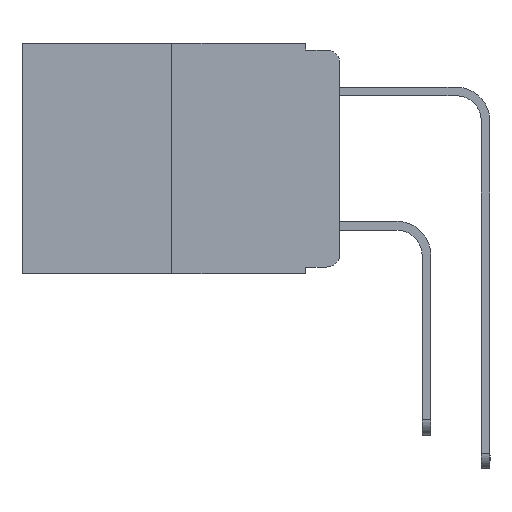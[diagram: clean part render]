
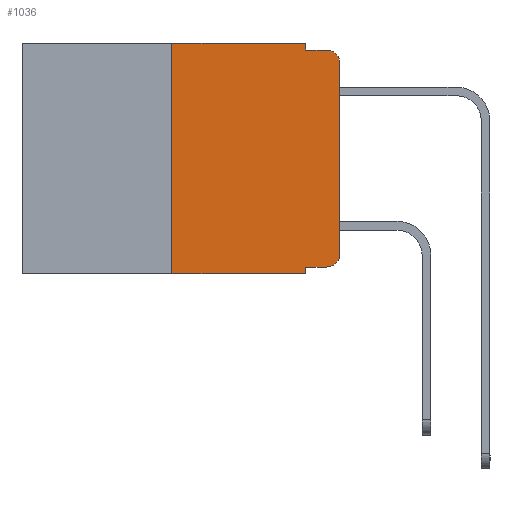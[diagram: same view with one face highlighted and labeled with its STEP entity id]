
A CAD part, left-side view. The second image highlights one B-rep face of the part: STEP entity #1036.
In plain terms, the highlighted planar face has unit normal (-1, 0, 0).
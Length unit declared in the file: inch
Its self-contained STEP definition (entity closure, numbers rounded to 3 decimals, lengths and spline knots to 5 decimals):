
#616 = ORIENTED_EDGE ( 'NONE', *, *, #22179, .F. ) ;
#884 = DIRECTION ( 'NONE',  ( 1., 0., 0. ) ) ;
#899 = LINE ( 'NONE', #18932, #20484 ) ;
#1036 = ADVANCED_FACE ( 'NONE', ( #2227 ), #2343, .F. ) ;
#1253 = DIRECTION ( 'NONE',  ( 0., -1., 0. ) ) ;
#1555 = ORIENTED_EDGE ( 'NONE', *, *, #3962, .F. ) ;
#1661 = CARTESIAN_POINT ( 'NONE',  ( 0., 0.473, 0. ) ) ;
#1679 = CARTESIAN_POINT ( 'NONE',  ( 0., 0., 0. ) ) ;
#1693 = CARTESIAN_POINT ( 'NONE',  ( 0., 0., -0.313 ) ) ;
#2227 = FACE_OUTER_BOUND ( 'NONE', #21097, .T. ) ;
#2343 = PLANE ( 'NONE',  #21999 ) ;
#2802 = CARTESIAN_POINT ( 'NONE',  ( 0., 0.051, -0.343 ) ) ;
#2828 = DIRECTION ( 'NONE',  ( 0., 0., -1. ) ) ;
#3444 = DIRECTION ( 'NONE',  ( 0., -1., 0. ) ) ;
#3516 = VERTEX_POINT ( 'NONE', #12894 ) ;
#3962 = EDGE_CURVE ( 'NONE', #21970, #14542, #13327, .T. ) ;
#4012 = LINE ( 'NONE', #13059, #9292 ) ;
#4331 = ORIENTED_EDGE ( 'NONE', *, *, #23583, .T. ) ;
#4602 = VERTEX_POINT ( 'NONE', #10375 ) ;
#4946 = EDGE_CURVE ( 'NONE', #21970, #4602, #16129, .T. ) ;
#5024 = ORIENTED_EDGE ( 'NONE', *, *, #16213, .T. ) ;
#5756 = DIRECTION ( 'NONE',  ( -1., 0., 0. ) ) ;
#6070 = ORIENTED_EDGE ( 'NONE', *, *, #4946, .T. ) ;
#6386 = ORIENTED_EDGE ( 'NONE', *, *, #7323, .F. ) ;
#6677 = ORIENTED_EDGE ( 'NONE', *, *, #18093, .T. ) ;
#6941 = CARTESIAN_POINT ( 'NONE',  ( 0., 0.051, -0.333 ) ) ;
#7323 = EDGE_CURVE ( 'NONE', #9462, #14646, #10969, .T. ) ;
#7603 = VERTEX_POINT ( 'NONE', #19814 ) ;
#8705 = AXIS2_PLACEMENT_3D ( 'NONE', #20191, #10854, #11677 ) ;
#9192 = CIRCLE ( 'NONE', #9973, 0.02 ) ;
#9292 = VECTOR ( 'NONE', #18643, 39.37008 ) ;
#9415 = EDGE_CURVE ( 'NONE', #18867, #9462, #4012, .T. ) ;
#9462 = VERTEX_POINT ( 'NONE', #16696 ) ;
#9466 = VECTOR ( 'NONE', #14877, 39.37008 ) ;
#9851 = CIRCLE ( 'NONE', #8705, 0.02 ) ;
#9973 = AXIS2_PLACEMENT_3D ( 'NONE', #12750, #5756, #20144 ) ;
#10375 = CARTESIAN_POINT ( 'NONE',  ( 0., 0.02, -0.333 ) ) ;
#10403 = CARTESIAN_POINT ( 'NONE',  ( 0., 0.051, 0. ) ) ;
#10482 = CARTESIAN_POINT ( 'NONE',  ( 0., 0.051, -0.333 ) ) ;
#10753 = DIRECTION ( 'NONE',  ( 0., 0., -1. ) ) ;
#10854 = DIRECTION ( 'NONE',  ( -1., 0., 0. ) ) ;
#10969 = LINE ( 'NONE', #1661, #20005 ) ;
#11475 = VERTEX_POINT ( 'NONE', #18108 ) ;
#11677 = DIRECTION ( 'NONE',  ( 0., 0., -1. ) ) ;
#12366 = CARTESIAN_POINT ( 'NONE',  ( 0., 0.25, -0.343 ) ) ;
#12536 = VERTEX_POINT ( 'NONE', #1693 ) ;
#12750 = CARTESIAN_POINT ( 'NONE',  ( 0., 0.02, -0.313 ) ) ;
#12894 = CARTESIAN_POINT ( 'NONE',  ( 0., 0.051, -0.01 ) ) ;
#12935 = LINE ( 'NONE', #1679, #9466 ) ;
#13059 = CARTESIAN_POINT ( 'NONE',  ( 0., 0.25, 0. ) ) ;
#13260 = VECTOR ( 'NONE', #10753, 39.37008 ) ;
#13327 = LINE ( 'NONE', #22907, #21570 ) ;
#13598 = DIRECTION ( 'NONE',  ( 0., -1., 0. ) ) ;
#14307 = VECTOR ( 'NONE', #3444, 39.37008 ) ;
#14542 = VERTEX_POINT ( 'NONE', #2802 ) ;
#14646 = VERTEX_POINT ( 'NONE', #10403 ) ;
#14796 = EDGE_CURVE ( 'NONE', #14646, #3516, #23851, .T. ) ;
#14877 = DIRECTION ( 'NONE',  ( 0., 0., 1. ) ) ;
#14930 = CARTESIAN_POINT ( 'NONE',  ( 0., 0.473, 0. ) ) ;
#16129 = LINE ( 'NONE', #6941, #22931 ) ;
#16213 = EDGE_CURVE ( 'NONE', #12536, #7603, #12935, .T. ) ;
#16426 = DIRECTION ( 'NONE',  ( 0., -1., 0. ) ) ;
#16696 = CARTESIAN_POINT ( 'NONE',  ( 0., 0.25, 0. ) ) ;
#16854 = ORIENTED_EDGE ( 'NONE', *, *, #14796, .F. ) ;
#18093 = EDGE_CURVE ( 'NONE', #7603, #11475, #9851, .T. ) ;
#18108 = CARTESIAN_POINT ( 'NONE',  ( 0., 0.02, -0.01 ) ) ;
#18643 = DIRECTION ( 'NONE',  ( 0., 0., 1. ) ) ;
#18867 = VERTEX_POINT ( 'NONE', #12366 ) ;
#18896 = DIRECTION ( 'NONE',  ( 0., 0., -1. ) ) ;
#18932 = CARTESIAN_POINT ( 'NONE',  ( 0., 0.051, -0.01 ) ) ;
#19814 = CARTESIAN_POINT ( 'NONE',  ( 0., 0., -0.03 ) ) ;
#20005 = VECTOR ( 'NONE', #16426, 39.37008 ) ;
#20144 = DIRECTION ( 'NONE',  ( 0., 0., -1. ) ) ;
#20191 = CARTESIAN_POINT ( 'NONE',  ( 0., 0.02, -0.03 ) ) ;
#20484 = VECTOR ( 'NONE', #13598, 39.37008 ) ;
#21083 = ORIENTED_EDGE ( 'NONE', *, *, #21549, .T. ) ;
#21097 = EDGE_LOOP ( 'NONE', ( #5024, #6677, #616, #16854, #6386, #21311, #4331, #1555, #6070, #21083 ) ) ;
#21311 = ORIENTED_EDGE ( 'NONE', *, *, #9415, .F. ) ;
#21549 = EDGE_CURVE ( 'NONE', #4602, #12536, #9192, .T. ) ;
#21570 = VECTOR ( 'NONE', #18896, 39.37008 ) ;
#21711 = LINE ( 'NONE', #23786, #14307 ) ;
#21970 = VERTEX_POINT ( 'NONE', #10482 ) ;
#21999 = AXIS2_PLACEMENT_3D ( 'NONE', #14930, #884, #2828 ) ;
#22179 = EDGE_CURVE ( 'NONE', #3516, #11475, #899, .T. ) ;
#22276 = CARTESIAN_POINT ( 'NONE',  ( 0., 0.051, 0. ) ) ;
#22907 = CARTESIAN_POINT ( 'NONE',  ( 0., 0.051, 0. ) ) ;
#22931 = VECTOR ( 'NONE', #1253, 39.37008 ) ;
#23583 = EDGE_CURVE ( 'NONE', #18867, #14542, #21711, .T. ) ;
#23786 = CARTESIAN_POINT ( 'NONE',  ( 0., 0.473, -0.343 ) ) ;
#23851 = LINE ( 'NONE', #22276, #13260 ) ;
